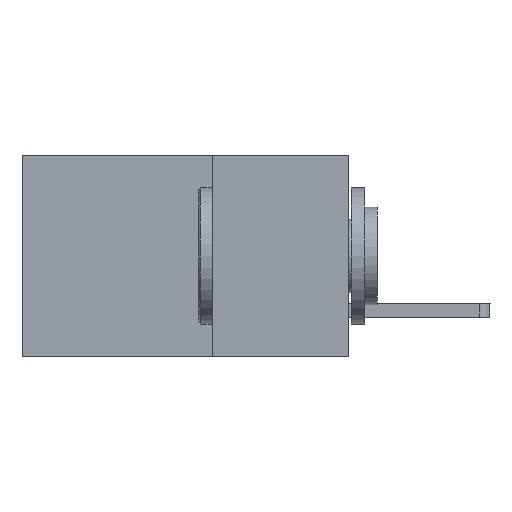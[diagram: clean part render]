
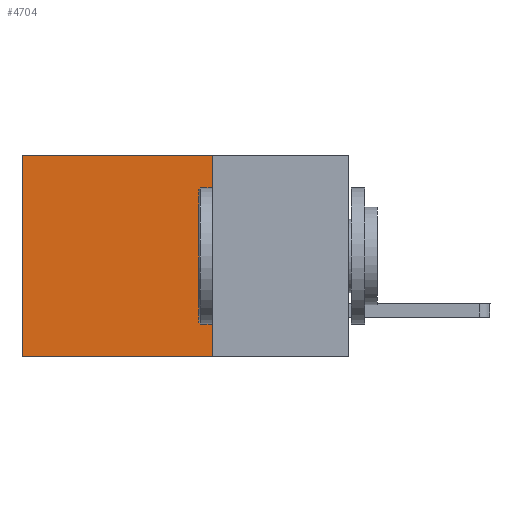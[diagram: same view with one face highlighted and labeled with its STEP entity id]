
A CAD part, left-side view. The second image highlights one B-rep face of the part: STEP entity #4704.
In plain terms, the highlighted planar face has unit normal (-1, 0, 0).
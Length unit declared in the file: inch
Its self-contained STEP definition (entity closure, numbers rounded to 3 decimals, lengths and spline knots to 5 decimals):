
#157 = EDGE_CURVE ( 'NONE', #498, #6011, #272, .T. ) ;
#272 = LINE ( 'NONE', #989, #3876 ) ;
#498 = VERTEX_POINT ( 'NONE', #6164 ) ;
#538 = ORIENTED_EDGE ( 'NONE', *, *, #5337, .T. ) ;
#602 = VERTEX_POINT ( 'NONE', #7035 ) ;
#810 = CARTESIAN_POINT ( 'NONE',  ( 0.2615, 0.6, -0.37 ) ) ;
#989 = CARTESIAN_POINT ( 'NONE',  ( 0.2615, 0.25, -0.37 ) ) ;
#998 = VERTEX_POINT ( 'NONE', #999 ) ;
#999 = CARTESIAN_POINT ( 'NONE',  ( 0.2615, 0.25, 0. ) ) ;
#1135 = EDGE_CURVE ( 'NONE', #998, #498, #3155, .T. ) ;
#1649 = DIRECTION ( 'NONE',  ( 1., 0., 0. ) ) ;
#1725 = ORIENTED_EDGE ( 'NONE', *, *, #157, .F. ) ;
#1875 = EDGE_CURVE ( 'NONE', #998, #602, #7764, .T. ) ;
#3018 = ORIENTED_EDGE ( 'NONE', *, *, #1135, .F. ) ;
#3152 = ORIENTED_EDGE ( 'NONE', *, *, #1875, .T. ) ;
#3155 = LINE ( 'NONE', #3913, #8246 ) ;
#3876 = VECTOR ( 'NONE', #5725, 39.37008 ) ;
#3913 = CARTESIAN_POINT ( 'NONE',  ( 0.2615, 0.25, -0.37 ) ) ;
#4426 = FACE_OUTER_BOUND ( 'NONE', #4725, .T. ) ;
#4704 = ADVANCED_FACE ( 'NONE', ( #4426 ), #6525, .F. ) ;
#4725 = EDGE_LOOP ( 'NONE', ( #538, #1725, #3018, #3152 ) ) ;
#5072 = CARTESIAN_POINT ( 'NONE',  ( 0.2615, 0.25, 0. ) ) ;
#5337 = EDGE_CURVE ( 'NONE', #602, #6011, #5720, .T. ) ;
#5720 = LINE ( 'NONE', #810, #8560 ) ;
#5725 = DIRECTION ( 'NONE',  ( 0., 1., 0. ) ) ;
#6011 = VERTEX_POINT ( 'NONE', #7254 ) ;
#6063 = VECTOR ( 'NONE', #8353, 39.37008 ) ;
#6164 = CARTESIAN_POINT ( 'NONE',  ( 0.2615, 0.25, -0.37 ) ) ;
#6409 = DIRECTION ( 'NONE',  ( 0., 0., -1. ) ) ;
#6525 = PLANE ( 'NONE',  #7539 ) ;
#6616 = CARTESIAN_POINT ( 'NONE',  ( 0.2615, 0.25, -0.37 ) ) ;
#7035 = CARTESIAN_POINT ( 'NONE',  ( 0.2615, 0.6, 0. ) ) ;
#7254 = CARTESIAN_POINT ( 'NONE',  ( 0.2615, 0.6, -0.37 ) ) ;
#7539 = AXIS2_PLACEMENT_3D ( 'NONE', #6616, #1649, #8648 ) ;
#7764 = LINE ( 'NONE', #5072, #6063 ) ;
#8246 = VECTOR ( 'NONE', #8730, 39.37008 ) ;
#8353 = DIRECTION ( 'NONE',  ( 0., 1., 0. ) ) ;
#8560 = VECTOR ( 'NONE', #6409, 39.37008 ) ;
#8648 = DIRECTION ( 'NONE',  ( 0., 0., -1. ) ) ;
#8730 = DIRECTION ( 'NONE',  ( 0., 0., -1. ) ) ;
